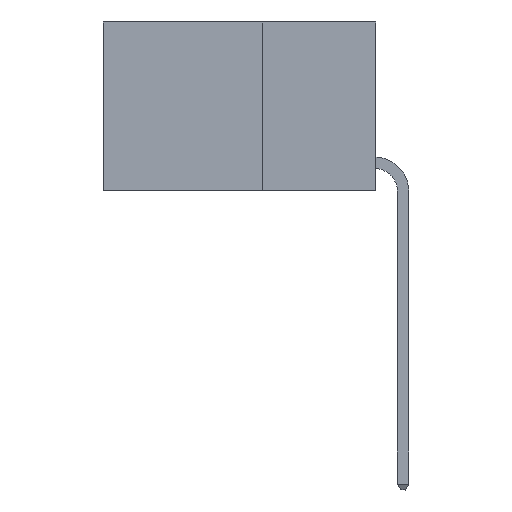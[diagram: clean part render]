
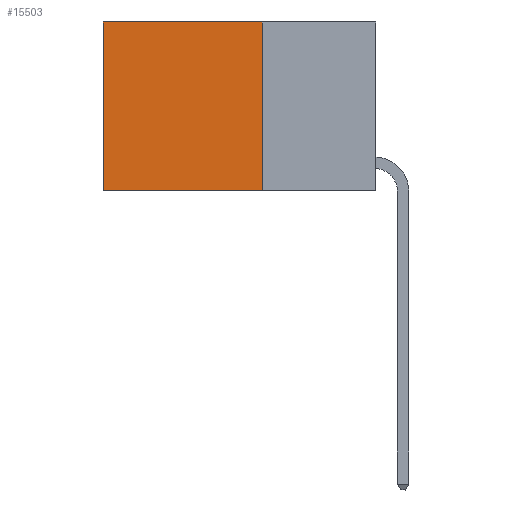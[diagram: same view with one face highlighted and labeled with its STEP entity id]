
A CAD part, left-side view. The second image highlights one B-rep face of the part: STEP entity #15503.
In plain terms, the highlighted planar face has unit normal (-1, 0, 0).
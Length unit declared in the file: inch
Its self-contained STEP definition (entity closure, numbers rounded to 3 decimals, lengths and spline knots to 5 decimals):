
#56 = VECTOR ( 'NONE', #22748, 39.37008 ) ;
#2438 = FACE_OUTER_BOUND ( 'NONE', #7931, .T. ) ;
#2844 = CARTESIAN_POINT ( 'NONE',  ( 0.2625, 0.25, 0. ) ) ;
#3068 = AXIS2_PLACEMENT_3D ( 'NONE', #18617, #6132, #20744 ) ;
#3161 = VERTEX_POINT ( 'NONE', #6644 ) ;
#4874 = ORIENTED_EDGE ( 'NONE', *, *, #11790, .T. ) ;
#5083 = VERTEX_POINT ( 'NONE', #10651 ) ;
#5730 = EDGE_CURVE ( 'NONE', #21033, #5083, #15895, .T. ) ;
#6026 = CARTESIAN_POINT ( 'NONE',  ( 0.2625, 0.6, 0. ) ) ;
#6132 = DIRECTION ( 'NONE',  ( 1., 0., 0. ) ) ;
#6279 = LINE ( 'NONE', #22318, #16706 ) ;
#6644 = CARTESIAN_POINT ( 'NONE',  ( 0.2625, 0.6, 0. ) ) ;
#7931 = EDGE_LOOP ( 'NONE', ( #26923, #14228, #19631, #4874 ) ) ;
#10651 = CARTESIAN_POINT ( 'NONE',  ( 0.2625, 0.25, -0.37 ) ) ;
#11790 = EDGE_CURVE ( 'NONE', #21033, #3161, #13941, .T. ) ;
#13297 = VECTOR ( 'NONE', #14783, 39.37008 ) ;
#13941 = LINE ( 'NONE', #14688, #13297 ) ;
#14037 = CARTESIAN_POINT ( 'NONE',  ( 0.2625, 0.25, 0. ) ) ;
#14228 = ORIENTED_EDGE ( 'NONE', *, *, #26867, .F. ) ;
#14387 = PLANE ( 'NONE',  #3068 ) ;
#14688 = CARTESIAN_POINT ( 'NONE',  ( 0.2625, 0.25, 0. ) ) ;
#14783 = DIRECTION ( 'NONE',  ( 0., 1., 0. ) ) ;
#15503 = ADVANCED_FACE ( 'NONE', ( #2438 ), #14387, .F. ) ;
#15895 = LINE ( 'NONE', #2844, #16007 ) ;
#16007 = VECTOR ( 'NONE', #17446, 39.37008 ) ;
#16706 = VECTOR ( 'NONE', #24420, 39.37008 ) ;
#16752 = VERTEX_POINT ( 'NONE', #26996 ) ;
#17388 = EDGE_CURVE ( 'NONE', #3161, #16752, #22338, .T. ) ;
#17446 = DIRECTION ( 'NONE',  ( 0., 0., -1. ) ) ;
#18617 = CARTESIAN_POINT ( 'NONE',  ( 0.2625, 0.25, 0. ) ) ;
#19631 = ORIENTED_EDGE ( 'NONE', *, *, #5730, .F. ) ;
#20744 = DIRECTION ( 'NONE',  ( 0., 0., -1. ) ) ;
#21033 = VERTEX_POINT ( 'NONE', #14037 ) ;
#22318 = CARTESIAN_POINT ( 'NONE',  ( 0.2625, 0.25, -0.37 ) ) ;
#22338 = LINE ( 'NONE', #6026, #56 ) ;
#22748 = DIRECTION ( 'NONE',  ( 0., 0., -1. ) ) ;
#24420 = DIRECTION ( 'NONE',  ( 0., 1., 0. ) ) ;
#26867 = EDGE_CURVE ( 'NONE', #5083, #16752, #6279, .T. ) ;
#26923 = ORIENTED_EDGE ( 'NONE', *, *, #17388, .T. ) ;
#26996 = CARTESIAN_POINT ( 'NONE',  ( 0.2625, 0.6, -0.37 ) ) ;
